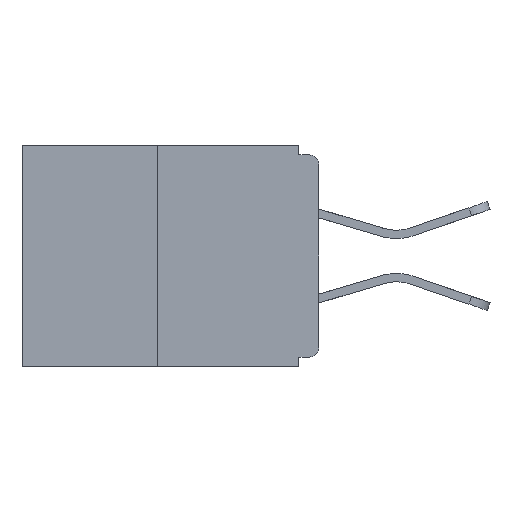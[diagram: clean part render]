
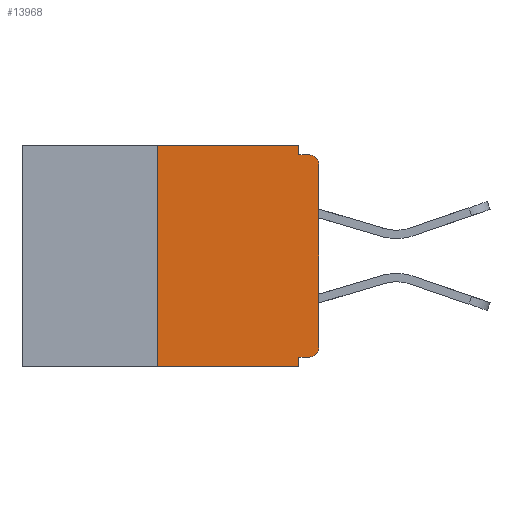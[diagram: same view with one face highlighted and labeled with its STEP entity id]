
A CAD part, left-side view. The second image highlights one B-rep face of the part: STEP entity #13968.
In plain terms, the highlighted planar face has unit normal (-1, 0, 0).
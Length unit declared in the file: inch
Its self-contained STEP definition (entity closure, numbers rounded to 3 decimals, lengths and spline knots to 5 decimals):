
#85 = VERTEX_POINT ( 'NONE', #19975 ) ;
#115 = VECTOR ( 'NONE', #14306, 39.37008 ) ;
#125 = DIRECTION ( 'NONE',  ( 0., -1., 0. ) ) ;
#214 = CARTESIAN_POINT ( 'NONE',  ( 0., 0.46, -0.343 ) ) ;
#221 = DIRECTION ( 'NONE',  ( 1., 0., 0. ) ) ;
#589 = CARTESIAN_POINT ( 'NONE',  ( 0., 0.25, 0. ) ) ;
#784 = EDGE_CURVE ( 'NONE', #13122, #7306, #11621, .T. ) ;
#1848 = CARTESIAN_POINT ( 'NONE',  ( 0., 0., 0. ) ) ;
#2435 = CIRCLE ( 'NONE', #15705, 0.015 ) ;
#3420 = EDGE_CURVE ( 'NONE', #16560, #9037, #21990, .T. ) ;
#3502 = ORIENTED_EDGE ( 'NONE', *, *, #22923, .F. ) ;
#4058 = CARTESIAN_POINT ( 'NONE',  ( 0., 0.25, 0. ) ) ;
#4436 = VECTOR ( 'NONE', #8569, 39.37008 ) ;
#4627 = DIRECTION ( 'NONE',  ( 0., 0., -1. ) ) ;
#4651 = CARTESIAN_POINT ( 'NONE',  ( 0., 0., -0.015 ) ) ;
#4726 = LINE ( 'NONE', #4651, #4436 ) ;
#4937 = DIRECTION ( 'NONE',  ( 0., -1., 0. ) ) ;
#5217 = LINE ( 'NONE', #11065, #12319 ) ;
#5391 = CARTESIAN_POINT ( 'NONE',  ( 0., 0.25, -0.343 ) ) ;
#5894 = CARTESIAN_POINT ( 'NONE',  ( 0., 0.031, 0. ) ) ;
#6340 = DIRECTION ( 'NONE',  ( -1., 0., 0. ) ) ;
#6764 = VERTEX_POINT ( 'NONE', #5894 ) ;
#6792 = FACE_OUTER_BOUND ( 'NONE', #20612, .T. ) ;
#7040 = ORIENTED_EDGE ( 'NONE', *, *, #15586, .F. ) ;
#7306 = VERTEX_POINT ( 'NONE', #23144 ) ;
#7369 = EDGE_CURVE ( 'NONE', #16560, #10461, #2435, .T. ) ;
#7777 = ORIENTED_EDGE ( 'NONE', *, *, #784, .T. ) ;
#8569 = DIRECTION ( 'NONE',  ( 0., -1., 0. ) ) ;
#8640 = ORIENTED_EDGE ( 'NONE', *, *, #3420, .F. ) ;
#8747 = CARTESIAN_POINT ( 'NONE',  ( 0., 0., -0.03 ) ) ;
#9037 = VERTEX_POINT ( 'NONE', #16873 ) ;
#9124 = ORIENTED_EDGE ( 'NONE', *, *, #23415, .T. ) ;
#9199 = VERTEX_POINT ( 'NONE', #5391 ) ;
#9206 = CARTESIAN_POINT ( 'NONE',  ( 0., 0., -0.313 ) ) ;
#9325 = DIRECTION ( 'NONE',  ( -1., 0., 0. ) ) ;
#9661 = LINE ( 'NONE', #214, #17271 ) ;
#10015 = PLANE ( 'NONE',  #11562 ) ;
#10461 = VERTEX_POINT ( 'NONE', #9206 ) ;
#10595 = DIRECTION ( 'NONE',  ( 0., 0., -1. ) ) ;
#10979 = CARTESIAN_POINT ( 'NONE',  ( 0., 0.46, 0. ) ) ;
#11065 = CARTESIAN_POINT ( 'NONE',  ( 0., 0.031, 0. ) ) ;
#11562 = AXIS2_PLACEMENT_3D ( 'NONE', #12004, #221, #10595 ) ;
#11621 = CIRCLE ( 'NONE', #22542, 0.015 ) ;
#11840 = EDGE_CURVE ( 'NONE', #14970, #6764, #24949, .T. ) ;
#12004 = CARTESIAN_POINT ( 'NONE',  ( 0., 0.46, 0. ) ) ;
#12022 = EDGE_CURVE ( 'NONE', #10461, #13122, #23109, .T. ) ;
#12040 = CARTESIAN_POINT ( 'NONE',  ( 0., 0.015, -0.313 ) ) ;
#12319 = VECTOR ( 'NONE', #15074, 39.37008 ) ;
#12408 = LINE ( 'NONE', #589, #115 ) ;
#13122 = VERTEX_POINT ( 'NONE', #8747 ) ;
#13332 = DIRECTION ( 'NONE',  ( 0., 0., -1. ) ) ;
#13544 = DIRECTION ( 'NONE',  ( 0., 1., 0. ) ) ;
#13804 = CARTESIAN_POINT ( 'NONE',  ( 0., 0., -0.328 ) ) ;
#13968 = ADVANCED_FACE ( 'NONE', ( #6792 ), #10015, .F. ) ;
#14094 = EDGE_CURVE ( 'NONE', #9037, #20530, #19891, .T. ) ;
#14306 = DIRECTION ( 'NONE',  ( 0., 0., 1. ) ) ;
#14970 = VERTEX_POINT ( 'NONE', #4058 ) ;
#15074 = DIRECTION ( 'NONE',  ( 0., 0., -1. ) ) ;
#15586 = EDGE_CURVE ( 'NONE', #9199, #14970, #12408, .T. ) ;
#15705 = AXIS2_PLACEMENT_3D ( 'NONE', #12040, #6340, #23979 ) ;
#16441 = ORIENTED_EDGE ( 'NONE', *, *, #7369, .T. ) ;
#16560 = VERTEX_POINT ( 'NONE', #21435 ) ;
#16873 = CARTESIAN_POINT ( 'NONE',  ( 0., 0.031, -0.328 ) ) ;
#16984 = CARTESIAN_POINT ( 'NONE',  ( 0., 0.015, -0.03 ) ) ;
#17079 = CARTESIAN_POINT ( 'NONE',  ( 0., 0.031, -0.343 ) ) ;
#17271 = VECTOR ( 'NONE', #125, 39.37008 ) ;
#17473 = ORIENTED_EDGE ( 'NONE', *, *, #17505, .F. ) ;
#17505 = EDGE_CURVE ( 'NONE', #6764, #85, #5217, .T. ) ;
#17523 = DIRECTION ( 'NONE',  ( 0., 0., 1. ) ) ;
#17909 = VECTOR ( 'NONE', #17523, 39.37008 ) ;
#18255 = ORIENTED_EDGE ( 'NONE', *, *, #14094, .F. ) ;
#19891 = LINE ( 'NONE', #22214, #23246 ) ;
#19975 = CARTESIAN_POINT ( 'NONE',  ( 0., 0.031, -0.015 ) ) ;
#20058 = VECTOR ( 'NONE', #4937, 39.37008 ) ;
#20530 = VERTEX_POINT ( 'NONE', #17079 ) ;
#20612 = EDGE_LOOP ( 'NONE', ( #23715, #7040, #9124, #18255, #8640, #16441, #24271, #7777, #3502, #17473 ) ) ;
#21435 = CARTESIAN_POINT ( 'NONE',  ( 0., 0.015, -0.328 ) ) ;
#21990 = LINE ( 'NONE', #13804, #23498 ) ;
#22214 = CARTESIAN_POINT ( 'NONE',  ( 0., 0.031, -0.343 ) ) ;
#22542 = AXIS2_PLACEMENT_3D ( 'NONE', #16984, #9325, #13332 ) ;
#22923 = EDGE_CURVE ( 'NONE', #85, #7306, #4726, .T. ) ;
#23109 = LINE ( 'NONE', #1848, #17909 ) ;
#23144 = CARTESIAN_POINT ( 'NONE',  ( 0., 0.015, -0.015 ) ) ;
#23246 = VECTOR ( 'NONE', #4627, 39.37008 ) ;
#23415 = EDGE_CURVE ( 'NONE', #9199, #20530, #9661, .T. ) ;
#23498 = VECTOR ( 'NONE', #13544, 39.37008 ) ;
#23715 = ORIENTED_EDGE ( 'NONE', *, *, #11840, .F. ) ;
#23979 = DIRECTION ( 'NONE',  ( 0., 0., -1. ) ) ;
#24271 = ORIENTED_EDGE ( 'NONE', *, *, #12022, .T. ) ;
#24949 = LINE ( 'NONE', #10979, #20058 ) ;
